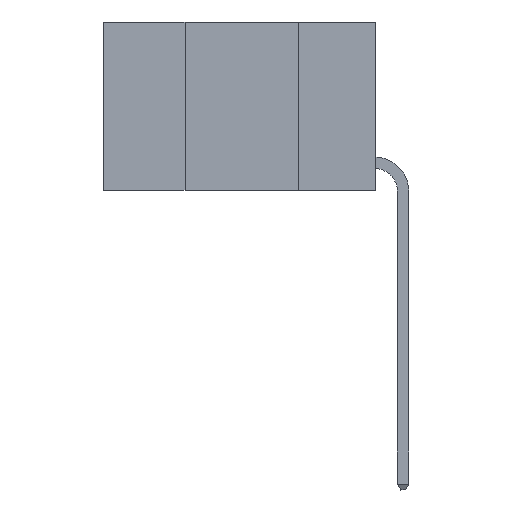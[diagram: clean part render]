
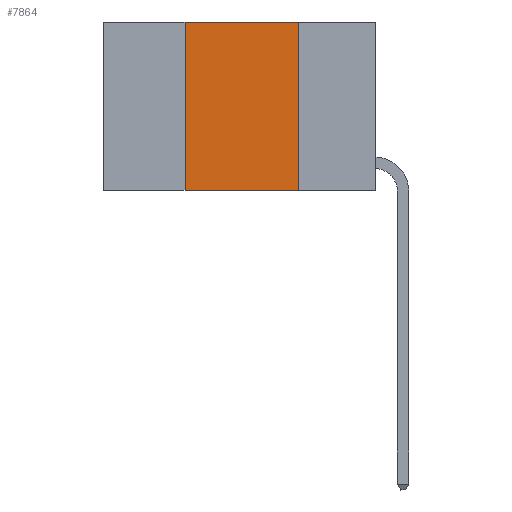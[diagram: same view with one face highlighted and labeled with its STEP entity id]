
A CAD part, left-side view. The second image highlights one B-rep face of the part: STEP entity #7864.
In plain terms, the highlighted planar face has unit normal (-1, 0, 0).
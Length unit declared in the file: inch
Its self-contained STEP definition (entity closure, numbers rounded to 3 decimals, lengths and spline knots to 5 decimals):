
#107 = ORIENTED_EDGE ( 'NONE', *, *, #1920, .F. ) ;
#333 = VERTEX_POINT ( 'NONE', #15184 ) ;
#829 = CARTESIAN_POINT ( 'NONE',  ( 0., 0.42, 0. ) ) ;
#1025 = EDGE_CURVE ( 'NONE', #333, #13334, #8558, .T. ) ;
#1920 = EDGE_CURVE ( 'NONE', #9836, #3012, #16000, .T. ) ;
#2601 = EDGE_CURVE ( 'NONE', #9836, #13334, #3275, .T. ) ;
#3012 = VERTEX_POINT ( 'NONE', #829 ) ;
#3275 = LINE ( 'NONE', #7262, #14778 ) ;
#3618 = DIRECTION ( 'NONE',  ( 0., 0., 1. ) ) ;
#3973 = AXIS2_PLACEMENT_3D ( 'NONE', #11505, #8020, #14178 ) ;
#3987 = LINE ( 'NONE', #8948, #11520 ) ;
#4768 = VECTOR ( 'NONE', #3618, 39.37008 ) ;
#4843 = CARTESIAN_POINT ( 'NONE',  ( 0., 0.42, 0. ) ) ;
#7262 = CARTESIAN_POINT ( 'NONE',  ( 0., 0.6, -0.37 ) ) ;
#7315 = VECTOR ( 'NONE', #8397, 39.37008 ) ;
#7319 = ORIENTED_EDGE ( 'NONE', *, *, #1025, .F. ) ;
#7864 = ADVANCED_FACE ( 'NONE', ( #10451 ), #15420, .F. ) ;
#7899 = ORIENTED_EDGE ( 'NONE', *, *, #2601, .T. ) ;
#8020 = DIRECTION ( 'NONE',  ( 1., 0., 0. ) ) ;
#8364 = ORIENTED_EDGE ( 'NONE', *, *, #8725, .F. ) ;
#8397 = DIRECTION ( 'NONE',  ( 0., 0., -1. ) ) ;
#8558 = LINE ( 'NONE', #15821, #7315 ) ;
#8725 = EDGE_CURVE ( 'NONE', #3012, #333, #3987, .T. ) ;
#8948 = CARTESIAN_POINT ( 'NONE',  ( 0., 0.6, 0. ) ) ;
#9836 = VERTEX_POINT ( 'NONE', #14654 ) ;
#10451 = FACE_OUTER_BOUND ( 'NONE', #15028, .T. ) ;
#10830 = DIRECTION ( 'NONE',  ( 0., -1., 0. ) ) ;
#11505 = CARTESIAN_POINT ( 'NONE',  ( 0., 0.6, 0. ) ) ;
#11520 = VECTOR ( 'NONE', #13891, 39.37008 ) ;
#13041 = CARTESIAN_POINT ( 'NONE',  ( 0., 0.17, -0.37 ) ) ;
#13334 = VERTEX_POINT ( 'NONE', #13041 ) ;
#13891 = DIRECTION ( 'NONE',  ( 0., -1., 0. ) ) ;
#14178 = DIRECTION ( 'NONE',  ( 0., 0., -1. ) ) ;
#14654 = CARTESIAN_POINT ( 'NONE',  ( 0., 0.42, -0.37 ) ) ;
#14778 = VECTOR ( 'NONE', #10830, 39.37008 ) ;
#15028 = EDGE_LOOP ( 'NONE', ( #7319, #8364, #107, #7899 ) ) ;
#15184 = CARTESIAN_POINT ( 'NONE',  ( 0., 0.17, 0. ) ) ;
#15420 = PLANE ( 'NONE',  #3973 ) ;
#15821 = CARTESIAN_POINT ( 'NONE',  ( 0., 0.17, 0. ) ) ;
#16000 = LINE ( 'NONE', #4843, #4768 ) ;
